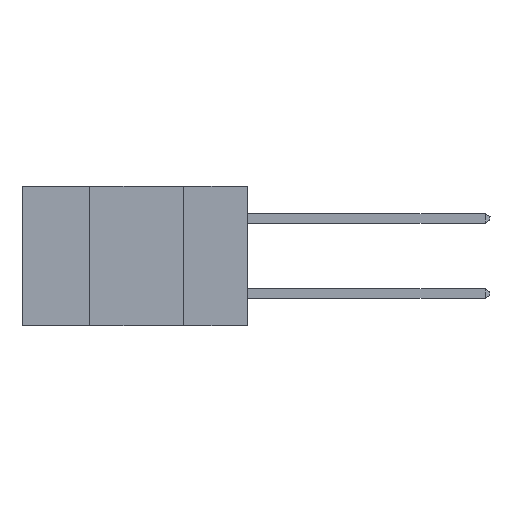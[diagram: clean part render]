
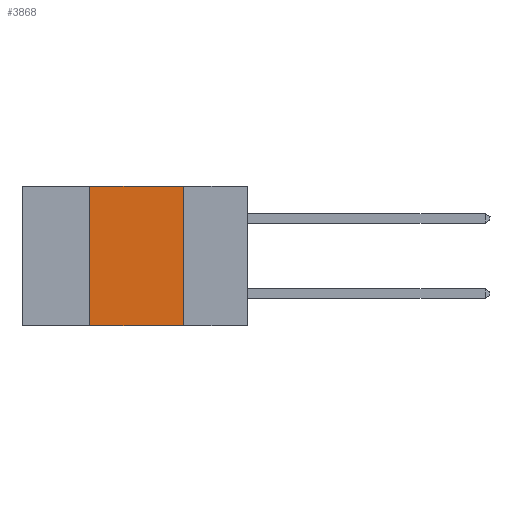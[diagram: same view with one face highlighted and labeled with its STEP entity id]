
A CAD part, left-side view. The second image highlights one B-rep face of the part: STEP entity #3868.
In plain terms, the highlighted planar face has unit normal (-1, 0, 0).
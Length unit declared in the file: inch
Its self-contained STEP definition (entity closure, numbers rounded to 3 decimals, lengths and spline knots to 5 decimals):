
#85 = DIRECTION ( 'NONE',  ( 0., 0., -1. ) ) ;
#514 = LINE ( 'NONE', #18469, #15761 ) ;
#1576 = CARTESIAN_POINT ( 'NONE',  ( 0., 0.6, 0. ) ) ;
#1705 = LINE ( 'NONE', #12157, #18695 ) ;
#3868 = ADVANCED_FACE ( 'NONE', ( #9263 ), #5817, .F. ) ;
#4142 = EDGE_CURVE ( 'NONE', #12167, #9031, #8279, .T. ) ;
#5817 = PLANE ( 'NONE',  #8383 ) ;
#5865 = CARTESIAN_POINT ( 'NONE',  ( 0., 0.42, 0. ) ) ;
#5985 = LINE ( 'NONE', #8660, #17139 ) ;
#7387 = DIRECTION ( 'NONE',  ( 0., 0., 1. ) ) ;
#7702 = ORIENTED_EDGE ( 'NONE', *, *, #15020, .F. ) ;
#7951 = ORIENTED_EDGE ( 'NONE', *, *, #4142, .F. ) ;
#8279 = LINE ( 'NONE', #12981, #17835 ) ;
#8383 = AXIS2_PLACEMENT_3D ( 'NONE', #1576, #11831, #85 ) ;
#8660 = CARTESIAN_POINT ( 'NONE',  ( 0., 0.6, -0.37 ) ) ;
#9031 = VERTEX_POINT ( 'NONE', #5865 ) ;
#9112 = EDGE_CURVE ( 'NONE', #15160, #10025, #514, .T. ) ;
#9263 = FACE_OUTER_BOUND ( 'NONE', #17155, .T. ) ;
#9492 = CARTESIAN_POINT ( 'NONE',  ( 0., 0.17, 0. ) ) ;
#9866 = ORIENTED_EDGE ( 'NONE', *, *, #17640, .T. ) ;
#9990 = CARTESIAN_POINT ( 'NONE',  ( 0., 0.17, -0.37 ) ) ;
#10025 = VERTEX_POINT ( 'NONE', #9990 ) ;
#11831 = DIRECTION ( 'NONE',  ( 1., 0., 0. ) ) ;
#12157 = CARTESIAN_POINT ( 'NONE',  ( 0., 0.6, 0. ) ) ;
#12167 = VERTEX_POINT ( 'NONE', #14485 ) ;
#12981 = CARTESIAN_POINT ( 'NONE',  ( 0., 0.42, -0.37 ) ) ;
#14485 = CARTESIAN_POINT ( 'NONE',  ( 0., 0.42, -0.37 ) ) ;
#15020 = EDGE_CURVE ( 'NONE', #9031, #15160, #1705, .T. ) ;
#15160 = VERTEX_POINT ( 'NONE', #9492 ) ;
#15219 = DIRECTION ( 'NONE',  ( 0., -1., 0. ) ) ;
#15761 = VECTOR ( 'NONE', #16911, 39.37008 ) ;
#16362 = DIRECTION ( 'NONE',  ( 0., -1., 0. ) ) ;
#16440 = ORIENTED_EDGE ( 'NONE', *, *, #9112, .F. ) ;
#16911 = DIRECTION ( 'NONE',  ( 0., 0., -1. ) ) ;
#17139 = VECTOR ( 'NONE', #16362, 39.37008 ) ;
#17155 = EDGE_LOOP ( 'NONE', ( #16440, #7702, #7951, #9866 ) ) ;
#17640 = EDGE_CURVE ( 'NONE', #12167, #10025, #5985, .T. ) ;
#17835 = VECTOR ( 'NONE', #7387, 39.37008 ) ;
#18469 = CARTESIAN_POINT ( 'NONE',  ( 0., 0.17, -0.37 ) ) ;
#18695 = VECTOR ( 'NONE', #15219, 39.37008 ) ;
